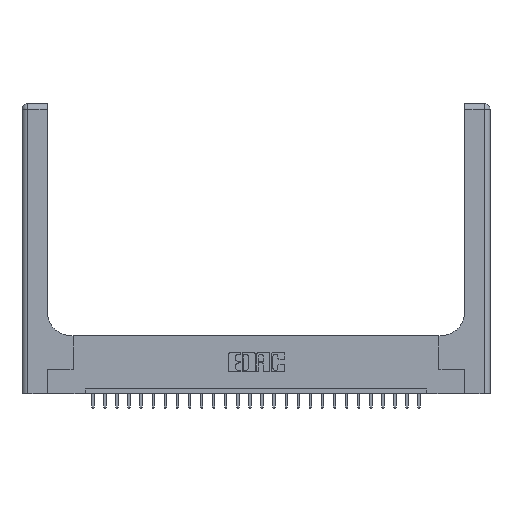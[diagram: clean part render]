
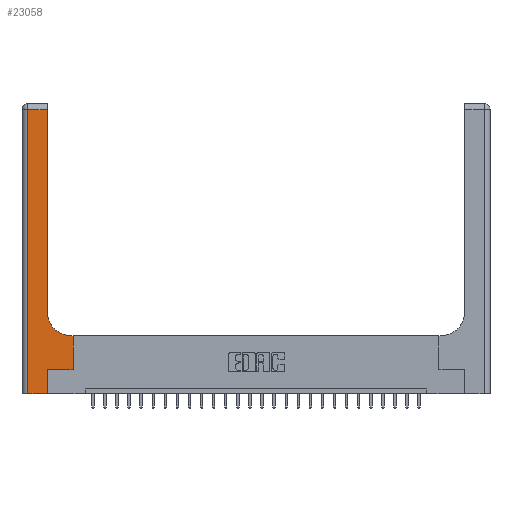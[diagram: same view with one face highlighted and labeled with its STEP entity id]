
A CAD part, top view. The second image highlights one B-rep face of the part: STEP entity #23058.
In plain terms, the highlighted planar face has unit normal (0, 0, 1).
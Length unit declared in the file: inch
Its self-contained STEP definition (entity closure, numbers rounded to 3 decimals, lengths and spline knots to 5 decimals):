
#373 = CARTESIAN_POINT ( 'NONE',  ( 0., 0., 0.37 ) ) ;
#1641 = DIRECTION ( 'NONE',  ( 0., 1., 0. ) ) ;
#1944 = FACE_OUTER_BOUND ( 'NONE', #16983, .T. ) ;
#2101 = EDGE_CURVE ( 'NONE', #7484, #5393, #7440, .T. ) ;
#2143 = CARTESIAN_POINT ( 'NONE',  ( 0.265, 0.25, 0.37 ) ) ;
#3139 = CARTESIAN_POINT ( 'NONE',  ( 0.26, 3., 0.37 ) ) ;
#3527 = LINE ( 'NONE', #10813, #10617 ) ;
#3932 = DIRECTION ( 'NONE',  ( 0., 0., -1. ) ) ;
#4344 = LINE ( 'NONE', #10566, #13774 ) ;
#5018 = DIRECTION ( 'NONE',  ( 0., 1., 0. ) ) ;
#5393 = VERTEX_POINT ( 'NONE', #17307 ) ;
#5408 = DIRECTION ( 'NONE',  ( -1., 0., 0. ) ) ;
#6062 = VERTEX_POINT ( 'NONE', #16877 ) ;
#6187 = EDGE_CURVE ( 'NONE', #10918, #13472, #23833, .T. ) ;
#6373 = VECTOR ( 'NONE', #11817, 39.37008 ) ;
#6648 = EDGE_CURVE ( 'NONE', #19250, #10918, #11347, .T. ) ;
#7034 = LINE ( 'NONE', #7594, #22126 ) ;
#7440 = LINE ( 'NONE', #10055, #18930 ) ;
#7484 = VERTEX_POINT ( 'NONE', #16092 ) ;
#7594 = CARTESIAN_POINT ( 'NONE',  ( 0.06, 3., 0.37 ) ) ;
#9159 = ORIENTED_EDGE ( 'NONE', *, *, #14815, .T. ) ;
#9466 = DIRECTION ( 'NONE',  ( 0., -1., 0. ) ) ;
#9475 = EDGE_CURVE ( 'NONE', #13472, #15925, #7034, .T. ) ;
#9580 = VECTOR ( 'NONE', #5018, 39.37008 ) ;
#9737 = CARTESIAN_POINT ( 'NONE',  ( 0., 2.94, 0.37 ) ) ;
#10055 = CARTESIAN_POINT ( 'NONE',  ( 0.26, 0.6, 0.37 ) ) ;
#10438 = DIRECTION ( 'NONE',  ( -1., 0., 0. ) ) ;
#10478 = VERTEX_POINT ( 'NONE', #19537 ) ;
#10566 = CARTESIAN_POINT ( 'NONE',  ( 0.265, 0., 0.37 ) ) ;
#10617 = VECTOR ( 'NONE', #1641, 39.37008 ) ;
#10813 = CARTESIAN_POINT ( 'NONE',  ( 0.528, 0.25, 0.37 ) ) ;
#10918 = VERTEX_POINT ( 'NONE', #22835 ) ;
#11347 = LINE ( 'NONE', #3139, #9580 ) ;
#11430 = CARTESIAN_POINT ( 'NONE',  ( 0.26, 0.85, 0.37 ) ) ;
#11817 = DIRECTION ( 'NONE',  ( 1., 0., 0. ) ) ;
#12367 = ORIENTED_EDGE ( 'NONE', *, *, #23591, .T. ) ;
#12523 = AXIS2_PLACEMENT_3D ( 'NONE', #13053, #20274, #12717 ) ;
#12541 = CIRCLE ( 'NONE', #12523, 0.25 ) ;
#12717 = DIRECTION ( 'NONE',  ( 1., 0., 0. ) ) ;
#12787 = ORIENTED_EDGE ( 'NONE', *, *, #19944, .T. ) ;
#13053 = CARTESIAN_POINT ( 'NONE',  ( 0.51, 0.85, 0.37 ) ) ;
#13472 = VERTEX_POINT ( 'NONE', #23183 ) ;
#13752 = ORIENTED_EDGE ( 'NONE', *, *, #2101, .T. ) ;
#13774 = VECTOR ( 'NONE', #17393, 39.37008 ) ;
#14248 = AXIS2_PLACEMENT_3D ( 'NONE', #22535, #3932, #16878 ) ;
#14815 = EDGE_CURVE ( 'NONE', #10478, #6062, #4344, .T. ) ;
#14981 = PLANE ( 'NONE',  #14248 ) ;
#15351 = DIRECTION ( 'NONE',  ( 1., 0., 0. ) ) ;
#15925 = VERTEX_POINT ( 'NONE', #23526 ) ;
#16009 = VECTOR ( 'NONE', #15351, 39.37008 ) ;
#16092 = CARTESIAN_POINT ( 'NONE',  ( 0.528, 0.6, 0.37 ) ) ;
#16823 = ORIENTED_EDGE ( 'NONE', *, *, #6187, .T. ) ;
#16829 = CARTESIAN_POINT ( 'NONE',  ( 0.528, 0.25, 0.37 ) ) ;
#16877 = CARTESIAN_POINT ( 'NONE',  ( 0.265, 0.25, 0.37 ) ) ;
#16878 = DIRECTION ( 'NONE',  ( -1., 0., 0. ) ) ;
#16983 = EDGE_LOOP ( 'NONE', ( #23957, #16823, #24386, #17112, #9159, #22334, #12787, #13752, #12367 ) ) ;
#17112 = ORIENTED_EDGE ( 'NONE', *, *, #23220, .T. ) ;
#17171 = LINE ( 'NONE', #2143, #16009 ) ;
#17307 = CARTESIAN_POINT ( 'NONE',  ( 0.51, 0.6, 0.37 ) ) ;
#17393 = DIRECTION ( 'NONE',  ( 0., 1., 0. ) ) ;
#17870 = EDGE_CURVE ( 'NONE', #6062, #20002, #17171, .T. ) ;
#18930 = VECTOR ( 'NONE', #5408, 39.37008 ) ;
#19250 = VERTEX_POINT ( 'NONE', #11430 ) ;
#19537 = CARTESIAN_POINT ( 'NONE',  ( 0.265, 0., 0.37 ) ) ;
#19944 = EDGE_CURVE ( 'NONE', #20002, #7484, #3527, .T. ) ;
#20002 = VERTEX_POINT ( 'NONE', #16829 ) ;
#20274 = DIRECTION ( 'NONE',  ( 0., 0., -1. ) ) ;
#21747 = VECTOR ( 'NONE', #10438, 39.37008 ) ;
#22126 = VECTOR ( 'NONE', #9466, 39.37008 ) ;
#22334 = ORIENTED_EDGE ( 'NONE', *, *, #17870, .T. ) ;
#22337 = LINE ( 'NONE', #373, #6373 ) ;
#22535 = CARTESIAN_POINT ( 'NONE',  ( 0., 3., 0.37 ) ) ;
#22835 = CARTESIAN_POINT ( 'NONE',  ( 0.26, 2.94, 0.37 ) ) ;
#23058 = ADVANCED_FACE ( 'NONE', ( #1944 ), #14981, .F. ) ;
#23183 = CARTESIAN_POINT ( 'NONE',  ( 0.06, 2.94, 0.37 ) ) ;
#23220 = EDGE_CURVE ( 'NONE', #15925, #10478, #22337, .T. ) ;
#23526 = CARTESIAN_POINT ( 'NONE',  ( 0.06, 0., 0.37 ) ) ;
#23591 = EDGE_CURVE ( 'NONE', #5393, #19250, #12541, .T. ) ;
#23833 = LINE ( 'NONE', #9737, #21747 ) ;
#23957 = ORIENTED_EDGE ( 'NONE', *, *, #6648, .T. ) ;
#24386 = ORIENTED_EDGE ( 'NONE', *, *, #9475, .T. ) ;
